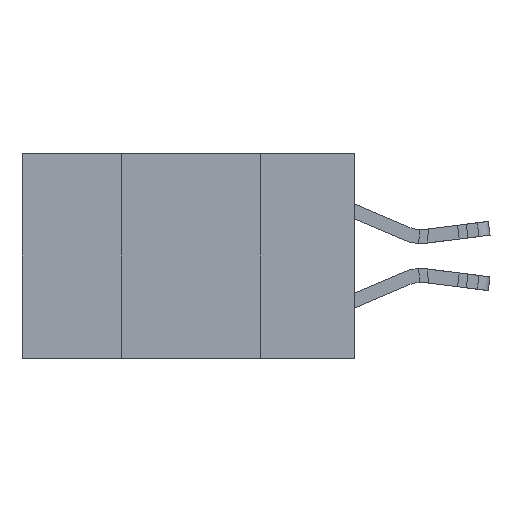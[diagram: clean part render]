
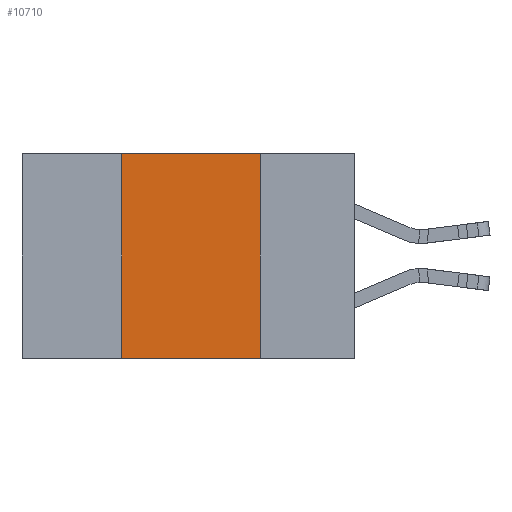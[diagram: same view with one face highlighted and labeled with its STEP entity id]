
A CAD part, left-side view. The second image highlights one B-rep face of the part: STEP entity #10710.
In plain terms, the highlighted planar face has unit normal (-1, 0, 0).
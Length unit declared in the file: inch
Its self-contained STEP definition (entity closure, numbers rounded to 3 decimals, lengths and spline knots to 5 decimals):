
#1709 = ORIENTED_EDGE ( 'NONE', *, *, #30862, .F. ) ;
#2451 = LINE ( 'NONE', #25633, #12528 ) ;
#5257 = CARTESIAN_POINT ( 'NONE',  ( 0., 0.42, 0. ) ) ;
#5953 = DIRECTION ( 'NONE',  ( 0., -1., 0. ) ) ;
#7218 = VERTEX_POINT ( 'NONE', #31296 ) ;
#7953 = CARTESIAN_POINT ( 'NONE',  ( 0., 0.6, 0. ) ) ;
#8145 = LINE ( 'NONE', #19443, #14034 ) ;
#9982 = DIRECTION ( 'NONE',  ( 1., 0., 0. ) ) ;
#10063 = VECTOR ( 'NONE', #10463, 39.37008 ) ;
#10463 = DIRECTION ( 'NONE',  ( 0., -1., 0. ) ) ;
#10710 = ADVANCED_FACE ( 'NONE', ( #16900 ), #22177, .F. ) ;
#11475 = DIRECTION ( 'NONE',  ( 0., 0., 1. ) ) ;
#12528 = VECTOR ( 'NONE', #5953, 39.37008 ) ;
#12845 = VERTEX_POINT ( 'NONE', #5257 ) ;
#14034 = VECTOR ( 'NONE', #19543, 39.37008 ) ;
#15796 = ORIENTED_EDGE ( 'NONE', *, *, #29116, .T. ) ;
#16900 = FACE_OUTER_BOUND ( 'NONE', #24029, .T. ) ;
#17206 = EDGE_CURVE ( 'NONE', #31147, #12845, #25499, .T. ) ;
#18356 = AXIS2_PLACEMENT_3D ( 'NONE', #24629, #9982, #27085 ) ;
#19214 = ORIENTED_EDGE ( 'NONE', *, *, #26091, .F. ) ;
#19443 = CARTESIAN_POINT ( 'NONE',  ( 0., 0.17, 0. ) ) ;
#19543 = DIRECTION ( 'NONE',  ( 0., 0., -1. ) ) ;
#20690 = ORIENTED_EDGE ( 'NONE', *, *, #17206, .F. ) ;
#21662 = CARTESIAN_POINT ( 'NONE',  ( 0., 0.17, -0.37 ) ) ;
#22177 = PLANE ( 'NONE',  #18356 ) ;
#23252 = CARTESIAN_POINT ( 'NONE',  ( 0., 0.42, -0.37 ) ) ;
#24029 = EDGE_LOOP ( 'NONE', ( #19214, #1709, #20690, #15796 ) ) ;
#24629 = CARTESIAN_POINT ( 'NONE',  ( 0., 0.6, 0. ) ) ;
#24739 = VECTOR ( 'NONE', #11475, 39.37008 ) ;
#25499 = LINE ( 'NONE', #26019, #24739 ) ;
#25633 = CARTESIAN_POINT ( 'NONE',  ( 0., 0.6, -0.37 ) ) ;
#26019 = CARTESIAN_POINT ( 'NONE',  ( 0., 0.42, 0. ) ) ;
#26091 = EDGE_CURVE ( 'NONE', #7218, #27256, #8145, .T. ) ;
#27085 = DIRECTION ( 'NONE',  ( 0., 0., -1. ) ) ;
#27256 = VERTEX_POINT ( 'NONE', #21662 ) ;
#29116 = EDGE_CURVE ( 'NONE', #31147, #27256, #2451, .T. ) ;
#29491 = LINE ( 'NONE', #7953, #10063 ) ;
#30862 = EDGE_CURVE ( 'NONE', #12845, #7218, #29491, .T. ) ;
#31147 = VERTEX_POINT ( 'NONE', #23252 ) ;
#31296 = CARTESIAN_POINT ( 'NONE',  ( 0., 0.17, 0. ) ) ;
